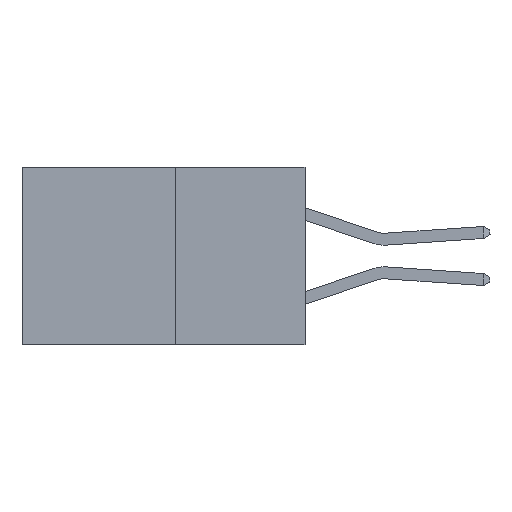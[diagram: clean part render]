
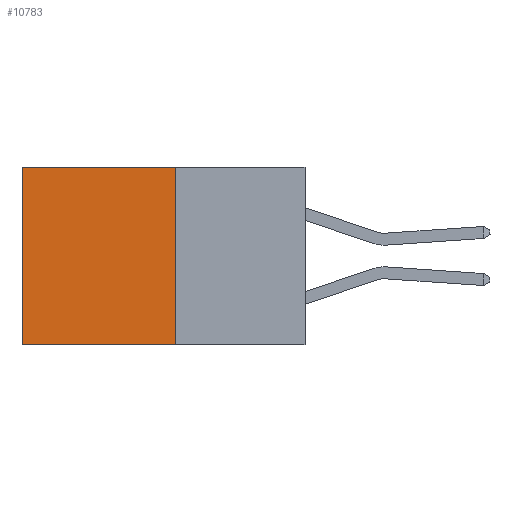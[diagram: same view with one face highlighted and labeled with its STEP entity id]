
A CAD part, left-side view. The second image highlights one B-rep face of the part: STEP entity #10783.
In plain terms, the highlighted planar face has unit normal (-1, 0, 0).
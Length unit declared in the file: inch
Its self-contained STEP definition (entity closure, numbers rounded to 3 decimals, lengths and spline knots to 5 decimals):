
#82 = LINE ( 'NONE', #18142, #7901 ) ;
#240 = CARTESIAN_POINT ( 'NONE',  ( 0.277, 0.27, -0.37 ) ) ;
#292 = CARTESIAN_POINT ( 'NONE',  ( 0.277, 0.27, 0. ) ) ;
#1294 = DIRECTION ( 'NONE',  ( 0., 1., 0. ) ) ;
#2001 = FACE_OUTER_BOUND ( 'NONE', #4168, .T. ) ;
#2380 = VERTEX_POINT ( 'NONE', #292 ) ;
#2572 = CARTESIAN_POINT ( 'NONE',  ( 0.277, 0.59, 0. ) ) ;
#3165 = EDGE_CURVE ( 'NONE', #2380, #5902, #11204, .T. ) ;
#3290 = AXIS2_PLACEMENT_3D ( 'NONE', #19844, #16623, #6780 ) ;
#3602 = DIRECTION ( 'NONE',  ( 0., 0., -1. ) ) ;
#3950 = LINE ( 'NONE', #240, #20928 ) ;
#3986 = ORIENTED_EDGE ( 'NONE', *, *, #14401, .T. ) ;
#4000 = VECTOR ( 'NONE', #1294, 39.37008 ) ;
#4168 = EDGE_LOOP ( 'NONE', ( #3986, #19707, #19274, #16192 ) ) ;
#5121 = PLANE ( 'NONE',  #3290 ) ;
#5902 = VERTEX_POINT ( 'NONE', #2572 ) ;
#6780 = DIRECTION ( 'NONE',  ( 0., 0., -1. ) ) ;
#7901 = VECTOR ( 'NONE', #11524, 39.37008 ) ;
#8083 = DIRECTION ( 'NONE',  ( 0., 0., -1. ) ) ;
#9439 = LINE ( 'NONE', #16198, #17676 ) ;
#10783 = ADVANCED_FACE ( 'NONE', ( #2001 ), #5121, .F. ) ;
#11204 = LINE ( 'NONE', #15163, #4000 ) ;
#11524 = DIRECTION ( 'NONE',  ( 0., 1., 0. ) ) ;
#12112 = CARTESIAN_POINT ( 'NONE',  ( 0.277, 0.27, -0.37 ) ) ;
#13878 = EDGE_CURVE ( 'NONE', #2380, #16015, #3950, .T. ) ;
#14401 = EDGE_CURVE ( 'NONE', #5902, #17855, #9439, .T. ) ;
#14499 = EDGE_CURVE ( 'NONE', #16015, #17855, #82, .T. ) ;
#15163 = CARTESIAN_POINT ( 'NONE',  ( 0.277, 0.27, 0. ) ) ;
#16015 = VERTEX_POINT ( 'NONE', #12112 ) ;
#16192 = ORIENTED_EDGE ( 'NONE', *, *, #3165, .T. ) ;
#16198 = CARTESIAN_POINT ( 'NONE',  ( 0.277, 0.59, -0.37 ) ) ;
#16623 = DIRECTION ( 'NONE',  ( 1., 0., 0. ) ) ;
#17676 = VECTOR ( 'NONE', #8083, 39.37008 ) ;
#17855 = VERTEX_POINT ( 'NONE', #19931 ) ;
#18142 = CARTESIAN_POINT ( 'NONE',  ( 0.277, 0.27, -0.37 ) ) ;
#19274 = ORIENTED_EDGE ( 'NONE', *, *, #13878, .F. ) ;
#19707 = ORIENTED_EDGE ( 'NONE', *, *, #14499, .F. ) ;
#19844 = CARTESIAN_POINT ( 'NONE',  ( 0.277, 0.27, -0.37 ) ) ;
#19931 = CARTESIAN_POINT ( 'NONE',  ( 0.277, 0.59, -0.37 ) ) ;
#20928 = VECTOR ( 'NONE', #3602, 39.37008 ) ;
